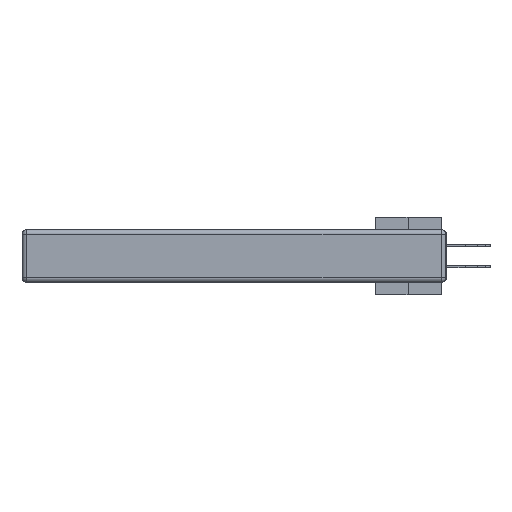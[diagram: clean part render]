
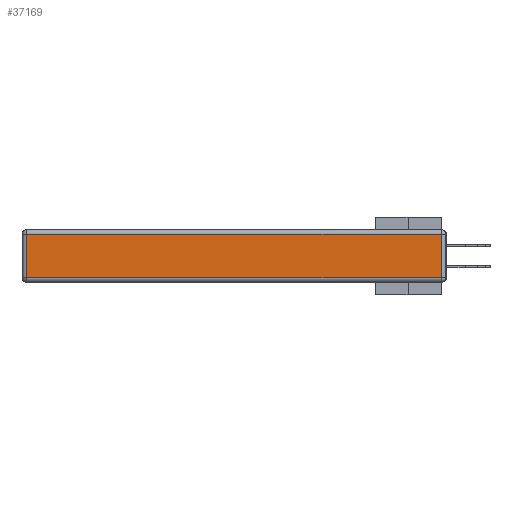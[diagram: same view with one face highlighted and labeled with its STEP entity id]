
A CAD part, left-side view. The second image highlights one B-rep face of the part: STEP entity #37169.
In plain terms, the highlighted planar face has unit normal (-1, 0, 0).
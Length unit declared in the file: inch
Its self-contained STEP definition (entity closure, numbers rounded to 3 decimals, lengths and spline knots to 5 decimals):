
#982 = LINE ( 'NONE', #21088, #19573 ) ;
#3322 = EDGE_LOOP ( 'NONE', ( #17635, #8720, #42124, #23908 ) ) ;
#3803 = EDGE_CURVE ( 'NONE', #40858, #24687, #982, .T. ) ;
#3998 = DIRECTION ( 'NONE',  ( 0., -1., 0. ) ) ;
#5328 = FACE_OUTER_BOUND ( 'NONE', #3322, .T. ) ;
#5468 = CARTESIAN_POINT ( 'NONE',  ( 0., 0.03, -0.343 ) ) ;
#7128 = VERTEX_POINT ( 'NONE', #44876 ) ;
#7992 = VECTOR ( 'NONE', #32352, 39.37008 ) ;
#8720 = ORIENTED_EDGE ( 'NONE', *, *, #39078, .T. ) ;
#9638 = DIRECTION ( 'NONE',  ( -1., 0., 0. ) ) ;
#11896 = CARTESIAN_POINT ( 'NONE',  ( 0., 0.03, -0.313 ) ) ;
#13144 = DIRECTION ( 'NONE',  ( 0., 0., 1. ) ) ;
#14929 = LINE ( 'NONE', #5468, #41304 ) ;
#17635 = ORIENTED_EDGE ( 'NONE', *, *, #3803, .T. ) ;
#18390 = LINE ( 'NONE', #24794, #7992 ) ;
#19573 = VECTOR ( 'NONE', #3998, 39.37008 ) ;
#20031 = PLANE ( 'NONE',  #37990 ) ;
#21088 = CARTESIAN_POINT ( 'NONE',  ( 0., 0., -0.313 ) ) ;
#23377 = VERTEX_POINT ( 'NONE', #32067 ) ;
#23551 = CARTESIAN_POINT ( 'NONE',  ( 0., 0., -0.343 ) ) ;
#23908 = ORIENTED_EDGE ( 'NONE', *, *, #31389, .T. ) ;
#24687 = VERTEX_POINT ( 'NONE', #11896 ) ;
#24794 = CARTESIAN_POINT ( 'NONE',  ( 0., 2.75, -0.03 ) ) ;
#25220 = DIRECTION ( 'NONE',  ( 0., 0., -1. ) ) ;
#25591 = LINE ( 'NONE', #35346, #42563 ) ;
#31389 = EDGE_CURVE ( 'NONE', #7128, #40858, #25591, .T. ) ;
#31824 = EDGE_CURVE ( 'NONE', #23377, #7128, #18390, .T. ) ;
#32067 = CARTESIAN_POINT ( 'NONE',  ( 0., 0.03, -0.03 ) ) ;
#32352 = DIRECTION ( 'NONE',  ( 0., 1., 0. ) ) ;
#33191 = DIRECTION ( 'NONE',  ( 0., 0., 1. ) ) ;
#35346 = CARTESIAN_POINT ( 'NONE',  ( 0., 2.72, -0.343 ) ) ;
#37169 = ADVANCED_FACE ( 'NONE', ( #5328 ), #20031, .T. ) ;
#37990 = AXIS2_PLACEMENT_3D ( 'NONE', #23551, #9638, #13144 ) ;
#39078 = EDGE_CURVE ( 'NONE', #24687, #23377, #14929, .T. ) ;
#40539 = CARTESIAN_POINT ( 'NONE',  ( 0., 2.72, -0.313 ) ) ;
#40858 = VERTEX_POINT ( 'NONE', #40539 ) ;
#41304 = VECTOR ( 'NONE', #33191, 39.37008 ) ;
#42124 = ORIENTED_EDGE ( 'NONE', *, *, #31824, .T. ) ;
#42563 = VECTOR ( 'NONE', #25220, 39.37008 ) ;
#44876 = CARTESIAN_POINT ( 'NONE',  ( 0., 2.72, -0.03 ) ) ;
